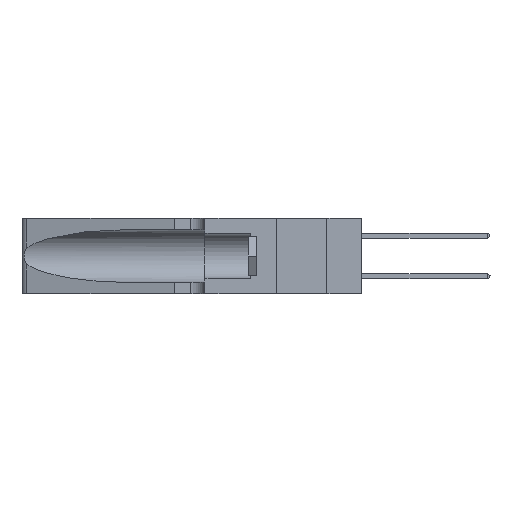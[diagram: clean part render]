
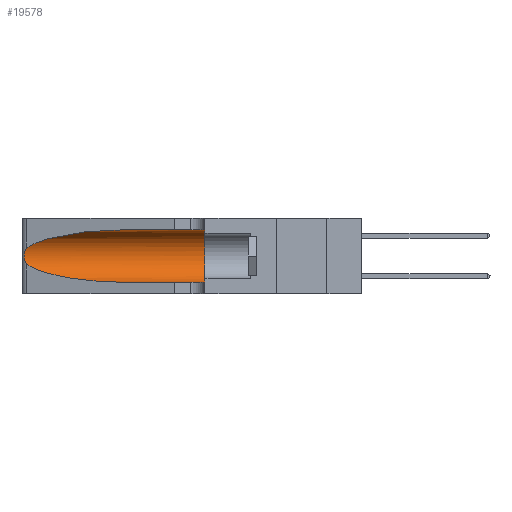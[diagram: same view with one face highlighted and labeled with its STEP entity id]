
A CAD part, left-side view. The second image highlights one B-rep face of the part: STEP entity #19578.
In plain terms, the highlighted cylindrical face has radius 3.308 mm (diameter 6.617 mm), a partial arc.
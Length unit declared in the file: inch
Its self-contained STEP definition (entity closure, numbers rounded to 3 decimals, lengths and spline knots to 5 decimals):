
#1593 = CARTESIAN_POINT ( 'NONE',  ( 0.1305, 1.61858, 0.05475 ) ) ;
#1810 = CARTESIAN_POINT ( 'NONE',  ( 0.1305, 1.61858, 0.31525 ) ) ;
#2150 = CARTESIAN_POINT ( 'NONE',  ( 0.1305, 0.72297, 0.31525 ) ) ;
#3049 = CARTESIAN_POINT ( 'NONE',  ( 0.25487, 1.22718, 0.22369 ) ) ;
#3147 = CARTESIAN_POINT ( 'NONE',  ( 0.18966, 0.96281, 0.31525 ) ) ;
#3469 = EDGE_CURVE ( 'NONE', #15122, #19015, #16193, .T. ) ;
#3786 = CARTESIAN_POINT ( 'NONE',  ( 0.1305, 0.72297, 0.05475 ) ) ;
#4074 = AXIS2_PLACEMENT_3D ( 'NONE', #12733, #19281, #8302 ) ;
#4810 = CARTESIAN_POINT ( 'NONE',  ( 0.25555, 1.22993, 0.14849 ) ) ;
#5078 = EDGE_CURVE ( 'NONE', #15122, #23705, #13590, .T. ) ;
#6683 = AXIS2_PLACEMENT_3D ( 'NONE', #25955, #14902, #17334 ) ;
#7013 = CARTESIAN_POINT ( 'NONE',  ( 0.25854, 1.2359, 0.20912 ) ) ;
#7113 = CARTESIAN_POINT ( 'NONE',  ( 0.25487, 1.22718, 0.22369 ) ) ;
#7123 = VERTEX_POINT ( 'NONE', #3786 ) ;
#7360 =( BOUNDED_CURVE ( )  B_SPLINE_CURVE ( 3, ( #24643, #11762, #26739, #18383 ),
 .UNSPECIFIED., .F., .T. ) 
 B_SPLINE_CURVE_WITH_KNOTS ( ( 4, 4 ),
 ( 3.44316, 4.71239 ),
 .UNSPECIFIED. ) 
 CURVE ( )  GEOMETRIC_REPRESENTATION_ITEM ( )  RATIONAL_B_SPLINE_CURVE ( ( 1., 0.87, 0.87, 1. ) ) 
 REPRESENTATION_ITEM ( '' )  );
#7673 = CARTESIAN_POINT ( 'NONE',  ( 0.1305, 0.35, 0.31525 ) ) ;
#8302 = DIRECTION ( 'NONE',  ( 0., 0., -1. ) ) ;
#9192 = CARTESIAN_POINT ( 'NONE',  ( 0.25639, 1.23186, 0.15144 ) ) ;
#9200 = VECTOR ( 'NONE', #12375, 39.37008 ) ;
#9281 = CARTESIAN_POINT ( 'NONE',  ( 0.25639, 1.23184, 0.21858 ) ) ;
#9704 = CARTESIAN_POINT ( 'NONE',  ( 0.2373, 1.15595, 0.28018 ) ) ;
#9731 = EDGE_CURVE ( 'NONE', #23705, #27143, #23855, .T. ) ;
#10343 = CYLINDRICAL_SURFACE ( 'NONE', #4074, 0.13025 ) ;
#10684 = CARTESIAN_POINT ( 'NONE',  ( 0.1305, 0.35, 0.05475 ) ) ;
#11348 = CARTESIAN_POINT ( 'NONE',  ( 0.25487, 1.22718, 0.14631 ) ) ;
#11451 = CARTESIAN_POINT ( 'NONE',  ( 0.25789, 1.23486, 0.15765 ) ) ;
#11632 = CARTESIAN_POINT ( 'NONE',  ( 0.26018, 1.23835, 0.19895 ) ) ;
#11762 = CARTESIAN_POINT ( 'NONE',  ( 0.2373, 1.15595, 0.08982 ) ) ;
#11888 = CARTESIAN_POINT ( 'NONE',  ( 0.1305, 0.72297, 0.31525 ) ) ;
#12023 = B_SPLINE_CURVE_WITH_KNOTS ( 'NONE', 3,
 ( #7113, #20341, #9281, #26520, #7013, #11632, #15719, #13815, #17983, #22140, #11451, #9192, #4810, #11348 ),
 .UNSPECIFIED., .F., .F.,
 ( 4, 2, 2, 2, 2, 2, 4 ),
 ( 0., 0.00027, 0.00053, 0.00107, 0.0016, 0.00187, 0.00214 ),
 .UNSPECIFIED. ) ;
#12375 = DIRECTION ( 'NONE',  ( 0., -1., 0. ) ) ;
#12733 = CARTESIAN_POINT ( 'NONE',  ( 0.1305, 1.61858, 0.185 ) ) ;
#12837 = ORIENTED_EDGE ( 'NONE', *, *, #3469, .T. ) ;
#13590 = LINE ( 'NONE', #1810, #9200 ) ;
#13815 = CARTESIAN_POINT ( 'NONE',  ( 0.26075, 1.23896, 0.178 ) ) ;
#14725 = VECTOR ( 'NONE', #16715, 39.37008 ) ;
#14902 = DIRECTION ( 'NONE',  ( 0., 1., 0. ) ) ;
#15122 = VERTEX_POINT ( 'NONE', #2150 ) ;
#15719 = CARTESIAN_POINT ( 'NONE',  ( 0.26075, 1.23896, 0.19203 ) ) ;
#16193 =( BOUNDED_CURVE ( )  B_SPLINE_CURVE ( 3, ( #11888, #3147, #9704, #3049 ),
 .UNSPECIFIED., .F., .F. ) 
 B_SPLINE_CURVE_WITH_KNOTS ( ( 4, 4 ),
 ( 1.5708, 2.84003 ),
 .UNSPECIFIED. ) 
 CURVE ( )  GEOMETRIC_REPRESENTATION_ITEM ( )  RATIONAL_B_SPLINE_CURVE ( ( 1., 0.87, 0.87, 1. ) ) 
 REPRESENTATION_ITEM ( '' )  );
#16715 = DIRECTION ( 'NONE',  ( 0., -1., 0. ) ) ;
#17334 = DIRECTION ( 'NONE',  ( 0., 0., 1. ) ) ;
#17393 = ORIENTED_EDGE ( 'NONE', *, *, #5078, .F. ) ;
#17983 = CARTESIAN_POINT ( 'NONE',  ( 0.26017, 1.23833, 0.17102 ) ) ;
#18278 = ORIENTED_EDGE ( 'NONE', *, *, #9731, .F. ) ;
#18383 = CARTESIAN_POINT ( 'NONE',  ( 0.1305, 0.72297, 0.05475 ) ) ;
#19015 = VERTEX_POINT ( 'NONE', #26106 ) ;
#19281 = DIRECTION ( 'NONE',  ( 0., -1., 0. ) ) ;
#19578 = ADVANCED_FACE ( 'NONE', ( #23917 ), #10343, .F. ) ;
#20266 = VERTEX_POINT ( 'NONE', #27790 ) ;
#20278 = EDGE_LOOP ( 'NONE', ( #12837, #20829, #27396, #27428, #18278, #17393 ) ) ;
#20341 = CARTESIAN_POINT ( 'NONE',  ( 0.25555, 1.22994, 0.2215 ) ) ;
#20829 = ORIENTED_EDGE ( 'NONE', *, *, #24050, .T. ) ;
#22140 = CARTESIAN_POINT ( 'NONE',  ( 0.25856, 1.23593, 0.16098 ) ) ;
#23705 = VERTEX_POINT ( 'NONE', #7673 ) ;
#23855 = CIRCLE ( 'NONE', #6683, 0.13025 ) ;
#23917 = FACE_OUTER_BOUND ( 'NONE', #20278, .T. ) ;
#24050 = EDGE_CURVE ( 'NONE', #19015, #20266, #12023, .T. ) ;
#24540 = LINE ( 'NONE', #1593, #14725 ) ;
#24643 = CARTESIAN_POINT ( 'NONE',  ( 0.25487, 1.22718, 0.14631 ) ) ;
#25004 = EDGE_CURVE ( 'NONE', #7123, #27143, #24540, .T. ) ;
#25433 = EDGE_CURVE ( 'NONE', #20266, #7123, #7360, .T. ) ;
#25955 = CARTESIAN_POINT ( 'NONE',  ( 0.1305, 0.35, 0.185 ) ) ;
#26106 = CARTESIAN_POINT ( 'NONE',  ( 0.25487, 1.22718, 0.22369 ) ) ;
#26520 = CARTESIAN_POINT ( 'NONE',  ( 0.25787, 1.23484, 0.2124 ) ) ;
#26739 = CARTESIAN_POINT ( 'NONE',  ( 0.18966, 0.96281, 0.05475 ) ) ;
#27143 = VERTEX_POINT ( 'NONE', #10684 ) ;
#27396 = ORIENTED_EDGE ( 'NONE', *, *, #25433, .T. ) ;
#27428 = ORIENTED_EDGE ( 'NONE', *, *, #25004, .T. ) ;
#27790 = CARTESIAN_POINT ( 'NONE',  ( 0.25487, 1.22718, 0.14631 ) ) ;
